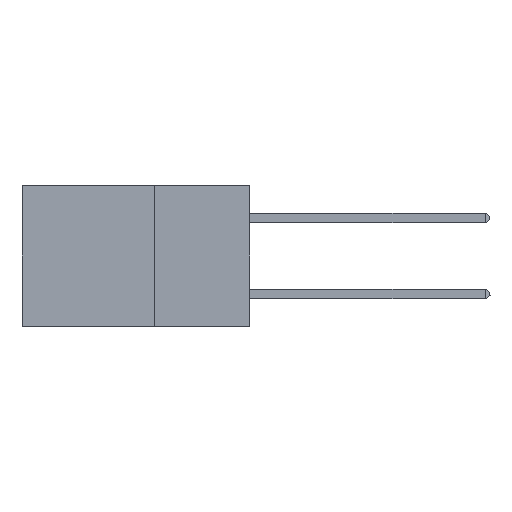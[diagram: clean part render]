
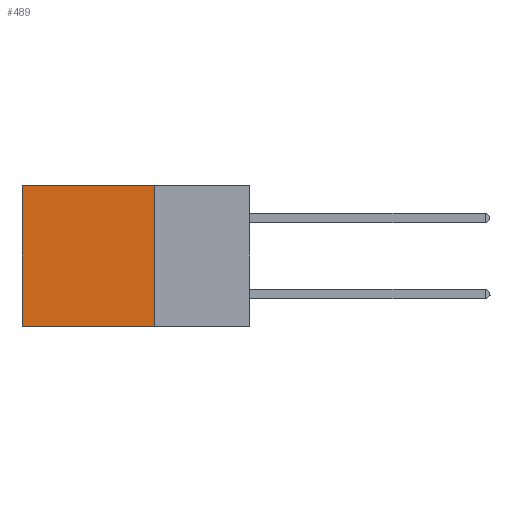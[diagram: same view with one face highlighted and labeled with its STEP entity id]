
A CAD part, left-side view. The second image highlights one B-rep face of the part: STEP entity #489.
In plain terms, the highlighted planar face has unit normal (-1, 0, 0).
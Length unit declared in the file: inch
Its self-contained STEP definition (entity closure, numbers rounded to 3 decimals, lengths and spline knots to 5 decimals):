
#489 = ADVANCED_FACE ( 'NONE', ( #11319 ), #1995, .F. ) ;
#773 = ORIENTED_EDGE ( 'NONE', *, *, #17030, .T. ) ;
#1174 = VERTEX_POINT ( 'NONE', #16002 ) ;
#1395 = DIRECTION ( 'NONE',  ( 0., 1., 0. ) ) ;
#1496 = LINE ( 'NONE', #2591, #14643 ) ;
#1995 = PLANE ( 'NONE',  #16318 ) ;
#2158 = VECTOR ( 'NONE', #12976, 39.37008 ) ;
#2591 = CARTESIAN_POINT ( 'NONE',  ( 0.2875, 0.25, -0.37 ) ) ;
#3251 = ORIENTED_EDGE ( 'NONE', *, *, #7339, .T. ) ;
#3319 = DIRECTION ( 'NONE',  ( 0., 0., -1. ) ) ;
#3642 = CARTESIAN_POINT ( 'NONE',  ( 0.2875, 0.6, 0. ) ) ;
#3933 = EDGE_LOOP ( 'NONE', ( #773, #13921, #4491, #3251 ) ) ;
#4491 = ORIENTED_EDGE ( 'NONE', *, *, #6249, .F. ) ;
#4765 = VERTEX_POINT ( 'NONE', #13083 ) ;
#6025 = CARTESIAN_POINT ( 'NONE',  ( 0.2875, 0.6, 0. ) ) ;
#6249 = EDGE_CURVE ( 'NONE', #4765, #1174, #11402, .T. ) ;
#7175 = CARTESIAN_POINT ( 'NONE',  ( 0.2875, 0.6, -0.37 ) ) ;
#7339 = EDGE_CURVE ( 'NONE', #4765, #13981, #12806, .T. ) ;
#7658 = VECTOR ( 'NONE', #10611, 39.37008 ) ;
#7868 = CARTESIAN_POINT ( 'NONE',  ( 0.2875, 0.25, 0. ) ) ;
#8268 = LINE ( 'NONE', #3642, #2158 ) ;
#9112 = CARTESIAN_POINT ( 'NONE',  ( 0.2875, 0.25, 0. ) ) ;
#10574 = VECTOR ( 'NONE', #15763, 39.37008 ) ;
#10611 = DIRECTION ( 'NONE',  ( 0., 1., 0. ) ) ;
#10746 = VERTEX_POINT ( 'NONE', #7175 ) ;
#11319 = FACE_OUTER_BOUND ( 'NONE', #3933, .T. ) ;
#11402 = LINE ( 'NONE', #7868, #10574 ) ;
#12806 = LINE ( 'NONE', #9112, #7658 ) ;
#12976 = DIRECTION ( 'NONE',  ( 0., 0., -1. ) ) ;
#13083 = CARTESIAN_POINT ( 'NONE',  ( 0.2875, 0.25, 0. ) ) ;
#13836 = CARTESIAN_POINT ( 'NONE',  ( 0.2875, 0.25, 0. ) ) ;
#13921 = ORIENTED_EDGE ( 'NONE', *, *, #14316, .F. ) ;
#13981 = VERTEX_POINT ( 'NONE', #6025 ) ;
#14316 = EDGE_CURVE ( 'NONE', #1174, #10746, #1496, .T. ) ;
#14643 = VECTOR ( 'NONE', #1395, 39.37008 ) ;
#15763 = DIRECTION ( 'NONE',  ( 0., 0., -1. ) ) ;
#16002 = CARTESIAN_POINT ( 'NONE',  ( 0.2875, 0.25, -0.37 ) ) ;
#16318 = AXIS2_PLACEMENT_3D ( 'NONE', #13836, #16544, #3319 ) ;
#16544 = DIRECTION ( 'NONE',  ( 1., 0., 0. ) ) ;
#17030 = EDGE_CURVE ( 'NONE', #13981, #10746, #8268, .T. ) ;
